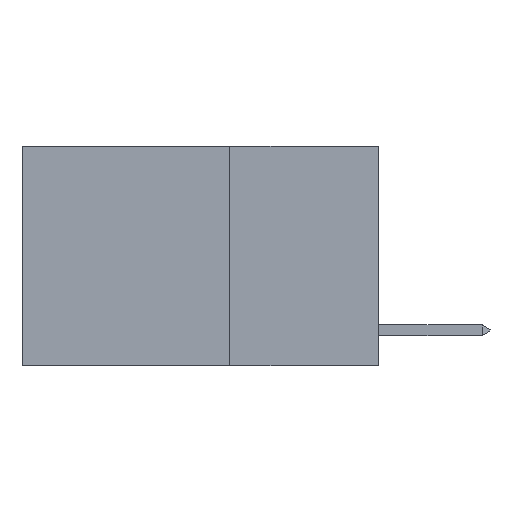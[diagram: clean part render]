
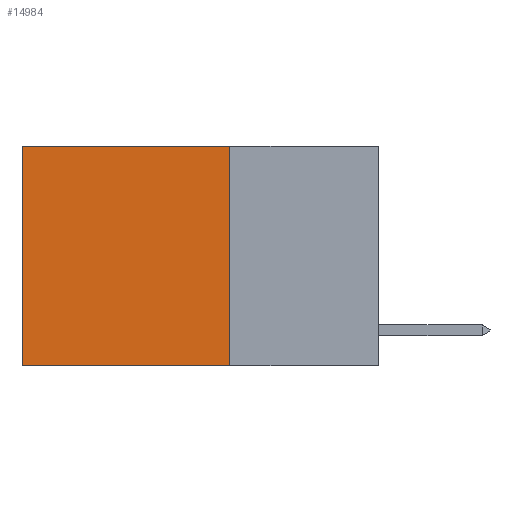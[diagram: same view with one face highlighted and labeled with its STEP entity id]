
A CAD part, left-side view. The second image highlights one B-rep face of the part: STEP entity #14984.
In plain terms, the highlighted planar face has unit normal (-1, 0, 0).
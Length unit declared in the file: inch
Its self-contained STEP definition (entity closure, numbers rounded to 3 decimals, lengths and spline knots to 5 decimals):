
#418 = AXIS2_PLACEMENT_3D ( 'NONE', #14167, #7724, #11251 ) ;
#981 = VECTOR ( 'NONE', #19037, 39.37008 ) ;
#1294 = CARTESIAN_POINT ( 'NONE',  ( 0.2625, 0.25, 0. ) ) ;
#2982 = PLANE ( 'NONE',  #418 ) ;
#3532 = EDGE_CURVE ( 'NONE', #20315, #8731, #18928, .T. ) ;
#3569 = ORIENTED_EDGE ( 'NONE', *, *, #5388, .F. ) ;
#5119 = DIRECTION ( 'NONE',  ( 0., 1., 0. ) ) ;
#5388 = EDGE_CURVE ( 'NONE', #8731, #18114, #17822, .T. ) ;
#6722 = EDGE_CURVE ( 'NONE', #20315, #16281, #16014, .T. ) ;
#7585 = DIRECTION ( 'NONE',  ( 0., 0., -1. ) ) ;
#7724 = DIRECTION ( 'NONE',  ( 1., 0., 0. ) ) ;
#8599 = ORIENTED_EDGE ( 'NONE', *, *, #3532, .F. ) ;
#8731 = VERTEX_POINT ( 'NONE', #14420 ) ;
#9953 = CARTESIAN_POINT ( 'NONE',  ( 0.2625, 0.25, -0.37 ) ) ;
#10393 = EDGE_LOOP ( 'NONE', ( #14434, #3569, #8599, #14405 ) ) ;
#11251 = DIRECTION ( 'NONE',  ( 0., 0., -1. ) ) ;
#13169 = VECTOR ( 'NONE', #5119, 39.37008 ) ;
#13186 = CARTESIAN_POINT ( 'NONE',  ( 0.2625, 0.25, 0. ) ) ;
#13301 = CARTESIAN_POINT ( 'NONE',  ( 0.2625, 0.25, 0. ) ) ;
#14073 = FACE_OUTER_BOUND ( 'NONE', #10393, .T. ) ;
#14167 = CARTESIAN_POINT ( 'NONE',  ( 0.2625, 0.25, 0. ) ) ;
#14405 = ORIENTED_EDGE ( 'NONE', *, *, #6722, .T. ) ;
#14420 = CARTESIAN_POINT ( 'NONE',  ( 0.2625, 0.25, -0.37 ) ) ;
#14434 = ORIENTED_EDGE ( 'NONE', *, *, #17577, .T. ) ;
#14984 = ADVANCED_FACE ( 'NONE', ( #14073 ), #2982, .F. ) ;
#16014 = LINE ( 'NONE', #13301, #13169 ) ;
#16065 = LINE ( 'NONE', #20818, #19680 ) ;
#16078 = DIRECTION ( 'NONE',  ( 0., 1., 0. ) ) ;
#16281 = VERTEX_POINT ( 'NONE', #18574 ) ;
#16862 = VECTOR ( 'NONE', #16078, 39.37008 ) ;
#17577 = EDGE_CURVE ( 'NONE', #16281, #18114, #16065, .T. ) ;
#17822 = LINE ( 'NONE', #9953, #16862 ) ;
#18114 = VERTEX_POINT ( 'NONE', #20895 ) ;
#18574 = CARTESIAN_POINT ( 'NONE',  ( 0.2625, 0.6, 0. ) ) ;
#18928 = LINE ( 'NONE', #1294, #981 ) ;
#19037 = DIRECTION ( 'NONE',  ( 0., 0., -1. ) ) ;
#19680 = VECTOR ( 'NONE', #7585, 39.37008 ) ;
#20315 = VERTEX_POINT ( 'NONE', #13186 ) ;
#20818 = CARTESIAN_POINT ( 'NONE',  ( 0.2625, 0.6, 0. ) ) ;
#20895 = CARTESIAN_POINT ( 'NONE',  ( 0.2625, 0.6, -0.37 ) ) ;
